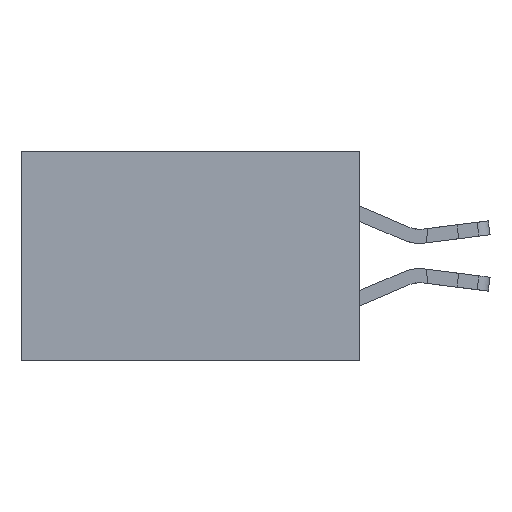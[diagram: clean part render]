
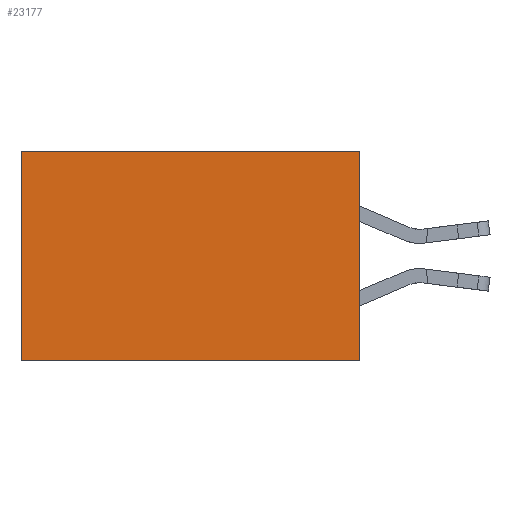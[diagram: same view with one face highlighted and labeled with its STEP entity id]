
A CAD part, left-side view. The second image highlights one B-rep face of the part: STEP entity #23177.
In plain terms, the highlighted planar face has unit normal (-1, 0, 0).
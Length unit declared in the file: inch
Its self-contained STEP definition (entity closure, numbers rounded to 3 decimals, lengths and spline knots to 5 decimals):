
#1095 = DIRECTION ( 'NONE',  ( 0., 0., -1. ) ) ;
#3208 = VERTEX_POINT ( 'NONE', #21659 ) ;
#3270 = VECTOR ( 'NONE', #24352, 39.37008 ) ;
#3582 = EDGE_CURVE ( 'NONE', #17395, #3208, #19859, .T. ) ;
#4977 = ORIENTED_EDGE ( 'NONE', *, *, #15996, .T. ) ;
#7540 = CARTESIAN_POINT ( 'NONE',  ( 0.2875, 0., 0. ) ) ;
#7623 = CARTESIAN_POINT ( 'NONE',  ( 0.2875, 0., 0. ) ) ;
#8942 = LINE ( 'NONE', #7623, #12200 ) ;
#9151 = EDGE_LOOP ( 'NONE', ( #27975, #19071, #11905, #4977 ) ) ;
#9531 = VECTOR ( 'NONE', #9864, 39.37008 ) ;
#9601 = CARTESIAN_POINT ( 'NONE',  ( 0.2875, 0.6, 0. ) ) ;
#9864 = DIRECTION ( 'NONE',  ( 0., 1., 0. ) ) ;
#10623 = CARTESIAN_POINT ( 'NONE',  ( 0.2875, 0., -0.37 ) ) ;
#11905 = ORIENTED_EDGE ( 'NONE', *, *, #24819, .F. ) ;
#12106 = VERTEX_POINT ( 'NONE', #29370 ) ;
#12200 = VECTOR ( 'NONE', #14352, 39.37008 ) ;
#12980 = DIRECTION ( 'NONE',  ( 0., 0., -1. ) ) ;
#13717 = AXIS2_PLACEMENT_3D ( 'NONE', #19870, #19967, #12980 ) ;
#14352 = DIRECTION ( 'NONE',  ( 0., 0., -1. ) ) ;
#14805 = CARTESIAN_POINT ( 'NONE',  ( 0.2875, 0.6, 0. ) ) ;
#14857 = VECTOR ( 'NONE', #1095, 39.37008 ) ;
#15996 = EDGE_CURVE ( 'NONE', #26826, #17395, #28614, .T. ) ;
#16961 = FACE_OUTER_BOUND ( 'NONE', #9151, .T. ) ;
#17395 = VERTEX_POINT ( 'NONE', #9601 ) ;
#18664 = LINE ( 'NONE', #10623, #3270 ) ;
#18692 = EDGE_CURVE ( 'NONE', #12106, #3208, #18664, .T. ) ;
#19071 = ORIENTED_EDGE ( 'NONE', *, *, #18692, .F. ) ;
#19859 = LINE ( 'NONE', #14805, #14857 ) ;
#19870 = CARTESIAN_POINT ( 'NONE',  ( 0.2875, 0., 0. ) ) ;
#19967 = DIRECTION ( 'NONE',  ( 1., 0., 0. ) ) ;
#20032 = CARTESIAN_POINT ( 'NONE',  ( 0.2875, 0., 0. ) ) ;
#21659 = CARTESIAN_POINT ( 'NONE',  ( 0.2875, 0.6, -0.37 ) ) ;
#23177 = ADVANCED_FACE ( 'NONE', ( #16961 ), #24676, .F. ) ;
#24352 = DIRECTION ( 'NONE',  ( 0., 1., 0. ) ) ;
#24676 = PLANE ( 'NONE',  #13717 ) ;
#24819 = EDGE_CURVE ( 'NONE', #26826, #12106, #8942, .T. ) ;
#26826 = VERTEX_POINT ( 'NONE', #20032 ) ;
#27975 = ORIENTED_EDGE ( 'NONE', *, *, #3582, .T. ) ;
#28614 = LINE ( 'NONE', #7540, #9531 ) ;
#29370 = CARTESIAN_POINT ( 'NONE',  ( 0.2875, 0., -0.37 ) ) ;
